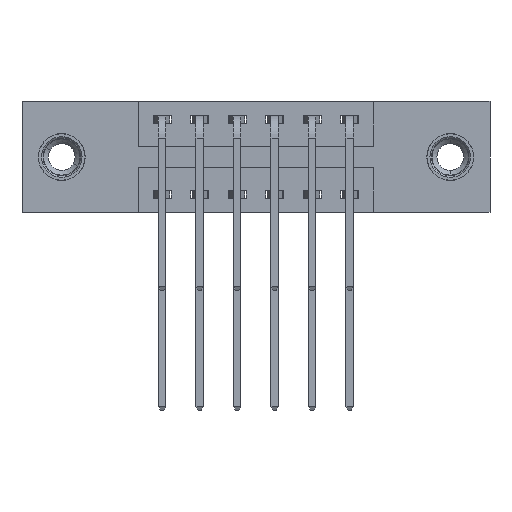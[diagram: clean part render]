
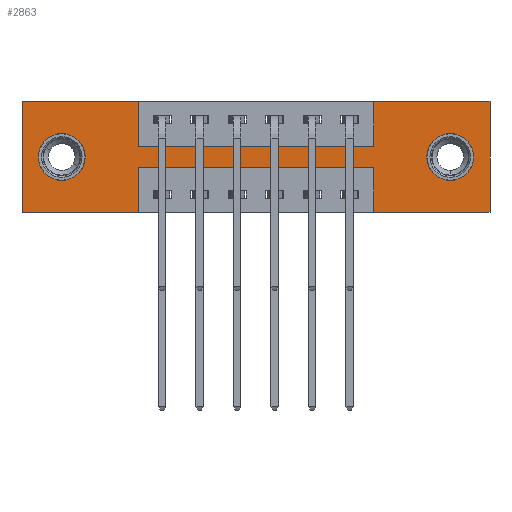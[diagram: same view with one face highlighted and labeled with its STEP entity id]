
A CAD part, front view. The second image highlights one B-rep face of the part: STEP entity #2863.
In plain terms, the highlighted planar face has unit normal (0, -1, 0).
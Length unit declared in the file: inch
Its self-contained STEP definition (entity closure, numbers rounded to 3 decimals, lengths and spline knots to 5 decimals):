
#53 = VERTEX_POINT ( 'NONE', #5109 ) ;
#67 = VECTOR ( 'NONE', #3888, 39.37008 ) ;
#137 = DIRECTION ( 'NONE',  ( 0., 1., 0. ) ) ;
#285 = CARTESIAN_POINT ( 'NONE',  ( 1.56, 0., 0. ) ) ;
#288 = VERTEX_POINT ( 'NONE', #7488 ) ;
#297 = EDGE_LOOP ( 'NONE', ( #2226, #2849 ) ) ;
#298 = DIRECTION ( 'NONE',  ( 0., 0., -1. ) ) ;
#344 = VECTOR ( 'NONE', #10736, 39.37008 ) ;
#471 = LINE ( 'NONE', #5322, #344 ) ;
#503 = CARTESIAN_POINT ( 'NONE',  ( 1.4275, 0., -0.263 ) ) ;
#557 = EDGE_CURVE ( 'NONE', #10824, #53, #6143, .T. ) ;
#664 = EDGE_CURVE ( 'NONE', #6428, #8626, #8390, .T. ) ;
#768 = EDGE_CURVE ( 'NONE', #5326, #8810, #1376, .T. ) ;
#813 = DIRECTION ( 'NONE',  ( 0., -1., 0. ) ) ;
#992 = EDGE_CURVE ( 'NONE', #1110, #6934, #8886, .T. ) ;
#1079 = DIRECTION ( 'NONE',  ( 0., 0., -1. ) ) ;
#1110 = VERTEX_POINT ( 'NONE', #5589 ) ;
#1351 = VECTOR ( 'NONE', #3730, 39.37008 ) ;
#1376 = CIRCLE ( 'NONE', #11505, 0.078 ) ;
#1461 = ORIENTED_EDGE ( 'NONE', *, *, #557, .F. ) ;
#1534 = DIRECTION ( 'NONE',  ( 1., 0., 0. ) ) ;
#1593 = ORIENTED_EDGE ( 'NONE', *, *, #9193, .F. ) ;
#1664 = EDGE_CURVE ( 'NONE', #288, #5833, #5745, .T. ) ;
#1707 = EDGE_CURVE ( 'NONE', #6231, #3996, #3727, .T. ) ;
#1773 = DIRECTION ( 'NONE',  ( -1., 0., 0. ) ) ;
#1838 = LINE ( 'NONE', #3608, #5351 ) ;
#1951 = ORIENTED_EDGE ( 'NONE', *, *, #9775, .F. ) ;
#2052 = VECTOR ( 'NONE', #298, 39.37008 ) ;
#2199 = AXIS2_PLACEMENT_3D ( 'NONE', #5304, #7045, #6208 ) ;
#2226 = ORIENTED_EDGE ( 'NONE', *, *, #1707, .T. ) ;
#2311 = VERTEX_POINT ( 'NONE', #7409 ) ;
#2318 = VECTOR ( 'NONE', #8687, 39.37008 ) ;
#2407 = ORIENTED_EDGE ( 'NONE', *, *, #664, .F. ) ;
#2429 = CARTESIAN_POINT ( 'NONE',  ( 0.3875, 0., -0.15 ) ) ;
#2441 = EDGE_CURVE ( 'NONE', #8810, #5326, #2859, .T. ) ;
#2557 = FACE_BOUND ( 'NONE', #297, .T. ) ;
#2561 = CARTESIAN_POINT ( 'NONE',  ( 1.4275, 0., -0.107 ) ) ;
#2772 = EDGE_CURVE ( 'NONE', #6934, #2311, #1838, .T. ) ;
#2849 = ORIENTED_EDGE ( 'NONE', *, *, #10629, .T. ) ;
#2859 = CIRCLE ( 'NONE', #2199, 0.078 ) ;
#2863 = ADVANCED_FACE ( 'NONE', ( #4931, #2557, #4611 ), #5346, .T. ) ;
#3127 = EDGE_CURVE ( 'NONE', #53, #6428, #9758, .T. ) ;
#3185 = CARTESIAN_POINT ( 'NONE',  ( 0.1325, 0., -0.185 ) ) ;
#3195 = ORIENTED_EDGE ( 'NONE', *, *, #3127, .F. ) ;
#3398 = AXIS2_PLACEMENT_3D ( 'NONE', #9441, #10366, #11292 ) ;
#3421 = EDGE_CURVE ( 'NONE', #8626, #7870, #6914, .T. ) ;
#3608 = CARTESIAN_POINT ( 'NONE',  ( 1.1725, 0., -0.37 ) ) ;
#3727 = CIRCLE ( 'NONE', #5285, 0.078 ) ;
#3730 = DIRECTION ( 'NONE',  ( 0., 0., 1. ) ) ;
#3794 = LINE ( 'NONE', #7687, #11359 ) ;
#3888 = DIRECTION ( 'NONE',  ( 0., 0., -1. ) ) ;
#3996 = VERTEX_POINT ( 'NONE', #4727 ) ;
#4121 = DIRECTION ( 'NONE',  ( 0., 0., 1. ) ) ;
#4280 = EDGE_CURVE ( 'NONE', #8353, #10323, #471, .T. ) ;
#4336 = ORIENTED_EDGE ( 'NONE', *, *, #768, .T. ) ;
#4495 = DIRECTION ( 'NONE',  ( 0., 0., -1. ) ) ;
#4611 = FACE_OUTER_BOUND ( 'NONE', #7620, .T. ) ;
#4723 = CARTESIAN_POINT ( 'NONE',  ( 0.3875, 0., -0.37 ) ) ;
#4727 = CARTESIAN_POINT ( 'NONE',  ( 0.1325, 0., -0.263 ) ) ;
#4764 = DIRECTION ( 'NONE',  ( 0., 0., -1. ) ) ;
#4931 = FACE_BOUND ( 'NONE', #9418, .T. ) ;
#4936 = ORIENTED_EDGE ( 'NONE', *, *, #9653, .F. ) ;
#5063 = CARTESIAN_POINT ( 'NONE',  ( 0.1325, 0., -0.107 ) ) ;
#5109 = CARTESIAN_POINT ( 'NONE',  ( 0., 0., 0. ) ) ;
#5285 = AXIS2_PLACEMENT_3D ( 'NONE', #3185, #6785, #8498 ) ;
#5304 = CARTESIAN_POINT ( 'NONE',  ( 1.4275, 0., -0.185 ) ) ;
#5322 = CARTESIAN_POINT ( 'NONE',  ( 0., 0., 0. ) ) ;
#5326 = VERTEX_POINT ( 'NONE', #503 ) ;
#5346 = PLANE ( 'NONE',  #7291 ) ;
#5351 = VECTOR ( 'NONE', #8131, 39.37008 ) ;
#5453 = DIRECTION ( 'NONE',  ( 1., 0., 0. ) ) ;
#5473 = VECTOR ( 'NONE', #1534, 39.37008 ) ;
#5589 = CARTESIAN_POINT ( 'NONE',  ( 1.56, 0., -0.37 ) ) ;
#5659 = CARTESIAN_POINT ( 'NONE',  ( 1.4275, 0., -0.185 ) ) ;
#5742 = DIRECTION ( 'NONE',  ( -1., 0., 0. ) ) ;
#5745 = LINE ( 'NONE', #4723, #11141 ) ;
#5833 = VERTEX_POINT ( 'NONE', #8920 ) ;
#5850 = CIRCLE ( 'NONE', #3398, 0.078 ) ;
#5978 = CARTESIAN_POINT ( 'NONE',  ( 0.3875, 0., -0.22 ) ) ;
#5985 = ORIENTED_EDGE ( 'NONE', *, *, #2772, .F. ) ;
#6143 = LINE ( 'NONE', #6187, #1351 ) ;
#6187 = CARTESIAN_POINT ( 'NONE',  ( 0., 0., 0. ) ) ;
#6208 = DIRECTION ( 'NONE',  ( 0., 0., -1. ) ) ;
#6231 = VERTEX_POINT ( 'NONE', #5063 ) ;
#6306 = CARTESIAN_POINT ( 'NONE',  ( 1.1725, 0., 0. ) ) ;
#6428 = VERTEX_POINT ( 'NONE', #6796 ) ;
#6488 = VECTOR ( 'NONE', #1773, 39.37008 ) ;
#6517 = ORIENTED_EDGE ( 'NONE', *, *, #992, .F. ) ;
#6573 = ORIENTED_EDGE ( 'NONE', *, *, #1664, .F. ) ;
#6785 = DIRECTION ( 'NONE',  ( 0., 1., 0. ) ) ;
#6796 = CARTESIAN_POINT ( 'NONE',  ( 0.3875, 0., 0. ) ) ;
#6914 = LINE ( 'NONE', #2429, #5473 ) ;
#6934 = VERTEX_POINT ( 'NONE', #8138 ) ;
#7045 = DIRECTION ( 'NONE',  ( 0., 1., 0. ) ) ;
#7087 = CARTESIAN_POINT ( 'NONE',  ( 1.1725, 0., -0.15 ) ) ;
#7291 = AXIS2_PLACEMENT_3D ( 'NONE', #8995, #813, #4495 ) ;
#7311 = LINE ( 'NONE', #11213, #67 ) ;
#7409 = CARTESIAN_POINT ( 'NONE',  ( 1.1725, 0., -0.22 ) ) ;
#7488 = CARTESIAN_POINT ( 'NONE',  ( 0.3875, 0., -0.22 ) ) ;
#7543 = CARTESIAN_POINT ( 'NONE',  ( 0., 0., -0.37 ) ) ;
#7620 = EDGE_LOOP ( 'NONE', ( #6573, #1593, #5985, #6517, #10033, #10459, #1951, #11257, #2407, #3195, #1461, #4936 ) ) ;
#7621 = EDGE_CURVE ( 'NONE', #10323, #1110, #7311, .T. ) ;
#7687 = CARTESIAN_POINT ( 'NONE',  ( 1.1725, 0., 0. ) ) ;
#7854 = CARTESIAN_POINT ( 'NONE',  ( 0., 0., 0. ) ) ;
#7870 = VERTEX_POINT ( 'NONE', #7087 ) ;
#8126 = CARTESIAN_POINT ( 'NONE',  ( 0., 0., -0.37 ) ) ;
#8131 = DIRECTION ( 'NONE',  ( 0., 0., 1. ) ) ;
#8138 = CARTESIAN_POINT ( 'NONE',  ( 1.1725, 0., -0.37 ) ) ;
#8353 = VERTEX_POINT ( 'NONE', #6306 ) ;
#8390 = LINE ( 'NONE', #11150, #2052 ) ;
#8424 = CARTESIAN_POINT ( 'NONE',  ( 0., 0., -0.37 ) ) ;
#8498 = DIRECTION ( 'NONE',  ( 0., 0., 1. ) ) ;
#8589 = VECTOR ( 'NONE', #5453, 39.37008 ) ;
#8612 = CARTESIAN_POINT ( 'NONE',  ( 0.3875, 0., -0.15 ) ) ;
#8626 = VERTEX_POINT ( 'NONE', #8612 ) ;
#8687 = DIRECTION ( 'NONE',  ( -1., 0., 0. ) ) ;
#8810 = VERTEX_POINT ( 'NONE', #2561 ) ;
#8886 = LINE ( 'NONE', #8126, #6488 ) ;
#8920 = CARTESIAN_POINT ( 'NONE',  ( 0.3875, 0., -0.37 ) ) ;
#8995 = CARTESIAN_POINT ( 'NONE',  ( 0., 0., -0.37 ) ) ;
#9193 = EDGE_CURVE ( 'NONE', #2311, #288, #10088, .T. ) ;
#9418 = EDGE_LOOP ( 'NONE', ( #9853, #4336 ) ) ;
#9441 = CARTESIAN_POINT ( 'NONE',  ( 0.1325, 0., -0.185 ) ) ;
#9653 = EDGE_CURVE ( 'NONE', #5833, #10824, #9920, .T. ) ;
#9758 = LINE ( 'NONE', #7854, #8589 ) ;
#9775 = EDGE_CURVE ( 'NONE', #7870, #8353, #3794, .T. ) ;
#9853 = ORIENTED_EDGE ( 'NONE', *, *, #2441, .T. ) ;
#9920 = LINE ( 'NONE', #8424, #10776 ) ;
#10033 = ORIENTED_EDGE ( 'NONE', *, *, #7621, .F. ) ;
#10088 = LINE ( 'NONE', #5978, #2318 ) ;
#10323 = VERTEX_POINT ( 'NONE', #285 ) ;
#10366 = DIRECTION ( 'NONE',  ( 0., 1., 0. ) ) ;
#10459 = ORIENTED_EDGE ( 'NONE', *, *, #4280, .F. ) ;
#10629 = EDGE_CURVE ( 'NONE', #3996, #6231, #5850, .T. ) ;
#10736 = DIRECTION ( 'NONE',  ( 1., 0., 0. ) ) ;
#10776 = VECTOR ( 'NONE', #5742, 39.37008 ) ;
#10824 = VERTEX_POINT ( 'NONE', #7543 ) ;
#11141 = VECTOR ( 'NONE', #4764, 39.37008 ) ;
#11150 = CARTESIAN_POINT ( 'NONE',  ( 0.3875, 0., 0. ) ) ;
#11213 = CARTESIAN_POINT ( 'NONE',  ( 1.56, 0., 0. ) ) ;
#11257 = ORIENTED_EDGE ( 'NONE', *, *, #3421, .F. ) ;
#11292 = DIRECTION ( 'NONE',  ( 0., 0., 1. ) ) ;
#11359 = VECTOR ( 'NONE', #4121, 39.37008 ) ;
#11505 = AXIS2_PLACEMENT_3D ( 'NONE', #5659, #137, #1079 ) ;
